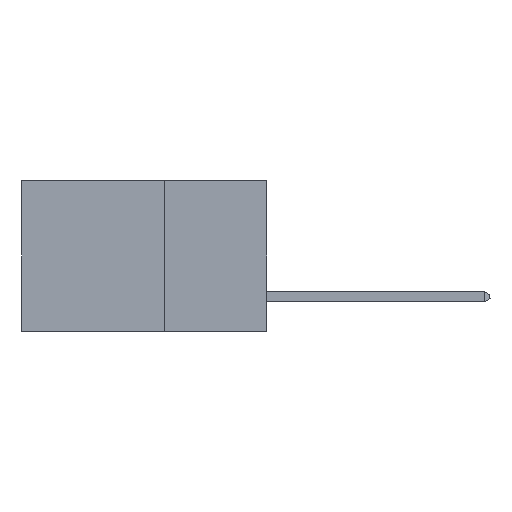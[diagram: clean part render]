
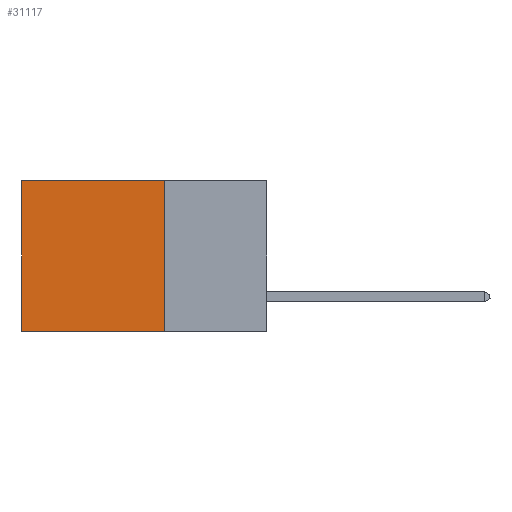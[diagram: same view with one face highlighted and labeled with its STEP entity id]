
A CAD part, left-side view. The second image highlights one B-rep face of the part: STEP entity #31117.
In plain terms, the highlighted planar face has unit normal (-1, 0, 0).
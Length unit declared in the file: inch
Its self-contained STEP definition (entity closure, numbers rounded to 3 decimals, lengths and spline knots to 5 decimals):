
#86 = LINE ( 'NONE', #23185, #15701 ) ;
#1261 = LINE ( 'NONE', #17314, #27144 ) ;
#1524 = LINE ( 'NONE', #12286, #27364 ) ;
#2162 = CARTESIAN_POINT ( 'NONE',  ( 0.2875, 0.25, -0.37 ) ) ;
#2337 = ORIENTED_EDGE ( 'NONE', *, *, #3945, .T. ) ;
#2440 = LINE ( 'NONE', #11676, #33257 ) ;
#3945 = EDGE_CURVE ( 'NONE', #8667, #24302, #2440, .T. ) ;
#6766 = CARTESIAN_POINT ( 'NONE',  ( 0.2875, 0.6, 0. ) ) ;
#6797 = CARTESIAN_POINT ( 'NONE',  ( 0.2875, 0.25, 0. ) ) ;
#7987 = EDGE_CURVE ( 'NONE', #12621, #24302, #86, .T. ) ;
#8227 = EDGE_LOOP ( 'NONE', ( #2337, #8232, #9399, #21649 ) ) ;
#8232 = ORIENTED_EDGE ( 'NONE', *, *, #7987, .F. ) ;
#8667 = VERTEX_POINT ( 'NONE', #6766 ) ;
#9399 = ORIENTED_EDGE ( 'NONE', *, *, #16765, .F. ) ;
#9708 = DIRECTION ( 'NONE',  ( 1., 0., 0. ) ) ;
#10612 = AXIS2_PLACEMENT_3D ( 'NONE', #6797, #9708, #14910 ) ;
#11676 = CARTESIAN_POINT ( 'NONE',  ( 0.2875, 0.6, 0. ) ) ;
#12054 = DIRECTION ( 'NONE',  ( 0., 0., -1. ) ) ;
#12286 = CARTESIAN_POINT ( 'NONE',  ( 0.2875, 0.25, 0. ) ) ;
#12621 = VERTEX_POINT ( 'NONE', #2162 ) ;
#14572 = CARTESIAN_POINT ( 'NONE',  ( 0.2875, 0.25, 0. ) ) ;
#14910 = DIRECTION ( 'NONE',  ( 0., 0., -1. ) ) ;
#15701 = VECTOR ( 'NONE', #28469, 39.37008 ) ;
#16765 = EDGE_CURVE ( 'NONE', #29934, #12621, #1261, .T. ) ;
#17186 = PLANE ( 'NONE',  #10612 ) ;
#17314 = CARTESIAN_POINT ( 'NONE',  ( 0.2875, 0.25, 0. ) ) ;
#19540 = EDGE_CURVE ( 'NONE', #29934, #8667, #1524, .T. ) ;
#21649 = ORIENTED_EDGE ( 'NONE', *, *, #19540, .T. ) ;
#23185 = CARTESIAN_POINT ( 'NONE',  ( 0.2875, 0.25, -0.37 ) ) ;
#23870 = CARTESIAN_POINT ( 'NONE',  ( 0.2875, 0.6, -0.37 ) ) ;
#24302 = VERTEX_POINT ( 'NONE', #23870 ) ;
#27144 = VECTOR ( 'NONE', #12054, 39.37008 ) ;
#27364 = VECTOR ( 'NONE', #32958, 39.37008 ) ;
#28469 = DIRECTION ( 'NONE',  ( 0., 1., 0. ) ) ;
#29934 = VERTEX_POINT ( 'NONE', #14572 ) ;
#31117 = ADVANCED_FACE ( 'NONE', ( #31169 ), #17186, .F. ) ;
#31169 = FACE_OUTER_BOUND ( 'NONE', #8227, .T. ) ;
#32784 = DIRECTION ( 'NONE',  ( 0., 0., -1. ) ) ;
#32958 = DIRECTION ( 'NONE',  ( 0., 1., 0. ) ) ;
#33257 = VECTOR ( 'NONE', #32784, 39.37008 ) ;
